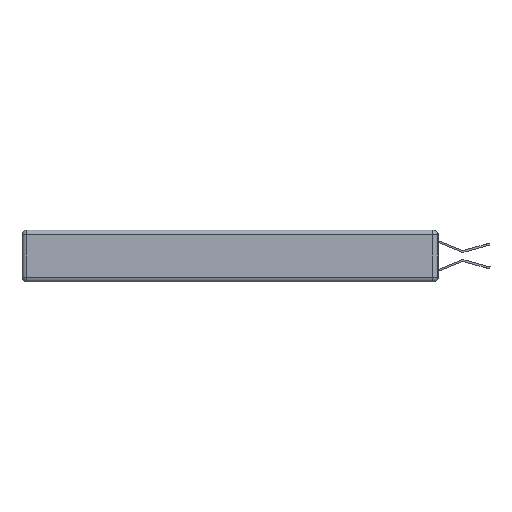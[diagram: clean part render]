
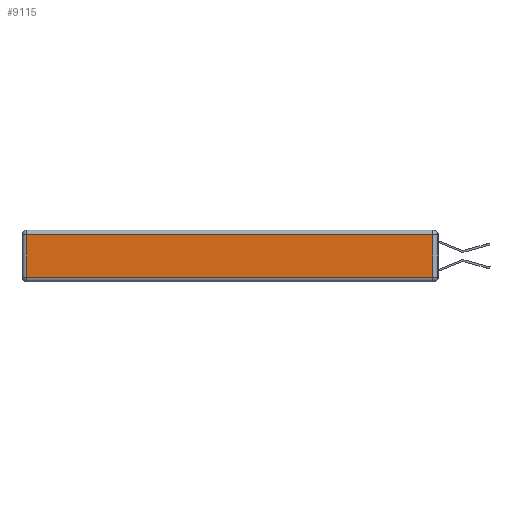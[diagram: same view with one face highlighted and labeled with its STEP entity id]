
A CAD part, left-side view. The second image highlights one B-rep face of the part: STEP entity #9115.
In plain terms, the highlighted planar face has unit normal (-1, 0, 0).
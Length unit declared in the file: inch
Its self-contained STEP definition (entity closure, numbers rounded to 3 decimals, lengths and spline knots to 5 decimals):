
#935 = EDGE_CURVE ( 'NONE', #5226, #2236, #10675, .T. ) ;
#2236 = VERTEX_POINT ( 'NONE', #2595 ) ;
#2595 = CARTESIAN_POINT ( 'NONE',  ( 0., 2.72, -0.03 ) ) ;
#2791 = AXIS2_PLACEMENT_3D ( 'NONE', #5156, #4100, #5252 ) ;
#2837 = PLANE ( 'NONE',  #2791 ) ;
#3009 = ORIENTED_EDGE ( 'NONE', *, *, #3962, .T. ) ;
#3062 = ORIENTED_EDGE ( 'NONE', *, *, #935, .T. ) ;
#3226 = CARTESIAN_POINT ( 'NONE',  ( 0., 0.03, -0.313 ) ) ;
#3259 = CARTESIAN_POINT ( 'NONE',  ( 0., 0.03, -0.03 ) ) ;
#3349 = CARTESIAN_POINT ( 'NONE',  ( 0., 2.75, -0.03 ) ) ;
#3893 = CARTESIAN_POINT ( 'NONE',  ( 0., 0.03, -0.343 ) ) ;
#3962 = EDGE_CURVE ( 'NONE', #10024, #5226, #12727, .T. ) ;
#4100 = DIRECTION ( 'NONE',  ( -1., 0., 0. ) ) ;
#4720 = LINE ( 'NONE', #12213, #9200 ) ;
#5156 = CARTESIAN_POINT ( 'NONE',  ( 0., 0., -0.343 ) ) ;
#5226 = VERTEX_POINT ( 'NONE', #3259 ) ;
#5252 = DIRECTION ( 'NONE',  ( 0., 0., 1. ) ) ;
#5297 = DIRECTION ( 'NONE',  ( 0., -1., 0. ) ) ;
#5741 = CARTESIAN_POINT ( 'NONE',  ( 0., 2.72, -0.343 ) ) ;
#5831 = DIRECTION ( 'NONE',  ( 0., 0., -1. ) ) ;
#6148 = DIRECTION ( 'NONE',  ( 0., 0., 1. ) ) ;
#6512 = CARTESIAN_POINT ( 'NONE',  ( 0., 2.72, -0.313 ) ) ;
#6909 = VECTOR ( 'NONE', #9008, 39.37008 ) ;
#7401 = EDGE_CURVE ( 'NONE', #9349, #10024, #4720, .T. ) ;
#7878 = ORIENTED_EDGE ( 'NONE', *, *, #7401, .T. ) ;
#8734 = EDGE_LOOP ( 'NONE', ( #7878, #3009, #3062, #14406 ) ) ;
#8904 = VECTOR ( 'NONE', #6148, 39.37008 ) ;
#9008 = DIRECTION ( 'NONE',  ( 0., 1., 0. ) ) ;
#9083 = LINE ( 'NONE', #5741, #14905 ) ;
#9115 = ADVANCED_FACE ( 'NONE', ( #13502 ), #2837, .T. ) ;
#9200 = VECTOR ( 'NONE', #5297, 39.37008 ) ;
#9349 = VERTEX_POINT ( 'NONE', #6512 ) ;
#10024 = VERTEX_POINT ( 'NONE', #3226 ) ;
#10675 = LINE ( 'NONE', #3349, #6909 ) ;
#11024 = EDGE_CURVE ( 'NONE', #2236, #9349, #9083, .T. ) ;
#12213 = CARTESIAN_POINT ( 'NONE',  ( 0., 0., -0.313 ) ) ;
#12727 = LINE ( 'NONE', #3893, #8904 ) ;
#13502 = FACE_OUTER_BOUND ( 'NONE', #8734, .T. ) ;
#14406 = ORIENTED_EDGE ( 'NONE', *, *, #11024, .T. ) ;
#14905 = VECTOR ( 'NONE', #5831, 39.37008 ) ;
